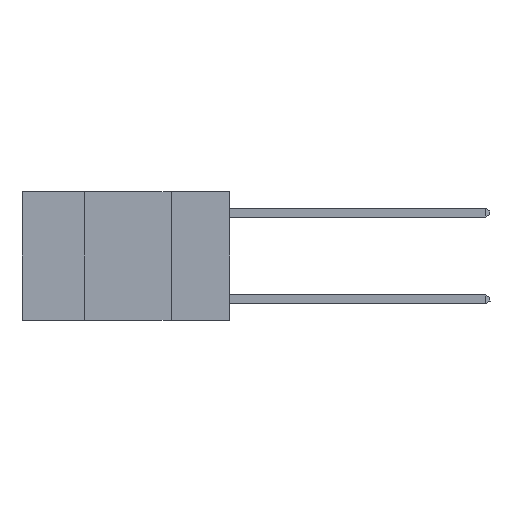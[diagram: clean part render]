
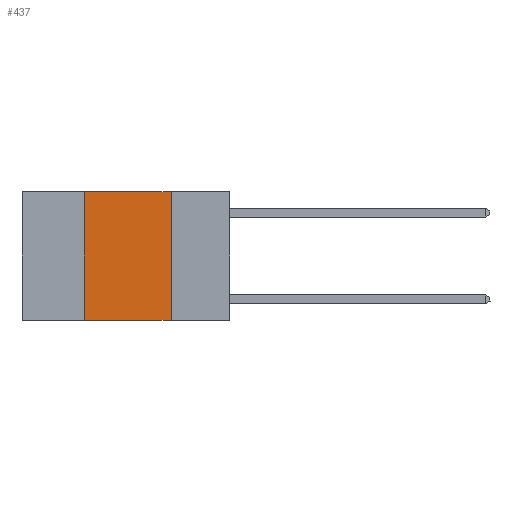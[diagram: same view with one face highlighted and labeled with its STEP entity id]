
A CAD part, left-side view. The second image highlights one B-rep face of the part: STEP entity #437.
In plain terms, the highlighted planar face has unit normal (-1, 0, 0).
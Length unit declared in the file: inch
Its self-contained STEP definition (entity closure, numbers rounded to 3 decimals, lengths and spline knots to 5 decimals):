
#437 = ADVANCED_FACE ( 'NONE', ( #4673 ), #18002, .F. ) ;
#825 = EDGE_CURVE ( 'NONE', #5001, #7185, #14611, .T. ) ;
#857 = CARTESIAN_POINT ( 'NONE',  ( 0., 0.6, 0. ) ) ;
#2220 = DIRECTION ( 'NONE',  ( 0., 0., 1. ) ) ;
#2278 = ORIENTED_EDGE ( 'NONE', *, *, #16851, .F. ) ;
#2785 = DIRECTION ( 'NONE',  ( 0., -1., 0. ) ) ;
#3053 = VECTOR ( 'NONE', #16009, 39.37008 ) ;
#4673 = FACE_OUTER_BOUND ( 'NONE', #8263, .T. ) ;
#4731 = LINE ( 'NONE', #10037, #11085 ) ;
#5001 = VERTEX_POINT ( 'NONE', #11899 ) ;
#6364 = VERTEX_POINT ( 'NONE', #7949 ) ;
#6952 = ORIENTED_EDGE ( 'NONE', *, *, #13907, .F. ) ;
#7185 = VERTEX_POINT ( 'NONE', #15652 ) ;
#7949 = CARTESIAN_POINT ( 'NONE',  ( 0., 0.42, -0.37 ) ) ;
#7953 = VECTOR ( 'NONE', #12514, 39.37008 ) ;
#8263 = EDGE_LOOP ( 'NONE', ( #9966, #6952, #2278, #13959 ) ) ;
#9477 = CARTESIAN_POINT ( 'NONE',  ( 0., 0.42, 0. ) ) ;
#9966 = ORIENTED_EDGE ( 'NONE', *, *, #825, .F. ) ;
#10037 = CARTESIAN_POINT ( 'NONE',  ( 0., 0.6, -0.37 ) ) ;
#11085 = VECTOR ( 'NONE', #2785, 39.37008 ) ;
#11437 = LINE ( 'NONE', #9477, #14397 ) ;
#11899 = CARTESIAN_POINT ( 'NONE',  ( 0., 0.17, 0. ) ) ;
#12131 = DIRECTION ( 'NONE',  ( 1., 0., 0. ) ) ;
#12514 = DIRECTION ( 'NONE',  ( 0., -1., 0. ) ) ;
#12975 = AXIS2_PLACEMENT_3D ( 'NONE', #16257, #12131, #16422 ) ;
#13907 = EDGE_CURVE ( 'NONE', #18645, #5001, #16570, .T. ) ;
#13959 = ORIENTED_EDGE ( 'NONE', *, *, #15091, .T. ) ;
#14397 = VECTOR ( 'NONE', #2220, 39.37008 ) ;
#14611 = LINE ( 'NONE', #15034, #3053 ) ;
#15034 = CARTESIAN_POINT ( 'NONE',  ( 0., 0.17, 0. ) ) ;
#15091 = EDGE_CURVE ( 'NONE', #6364, #7185, #4731, .T. ) ;
#15652 = CARTESIAN_POINT ( 'NONE',  ( 0., 0.17, -0.37 ) ) ;
#16009 = DIRECTION ( 'NONE',  ( 0., 0., -1. ) ) ;
#16257 = CARTESIAN_POINT ( 'NONE',  ( 0., 0.6, 0. ) ) ;
#16422 = DIRECTION ( 'NONE',  ( 0., 0., -1. ) ) ;
#16570 = LINE ( 'NONE', #857, #7953 ) ;
#16851 = EDGE_CURVE ( 'NONE', #6364, #18645, #11437, .T. ) ;
#17817 = CARTESIAN_POINT ( 'NONE',  ( 0., 0.42, 0. ) ) ;
#18002 = PLANE ( 'NONE',  #12975 ) ;
#18645 = VERTEX_POINT ( 'NONE', #17817 ) ;
